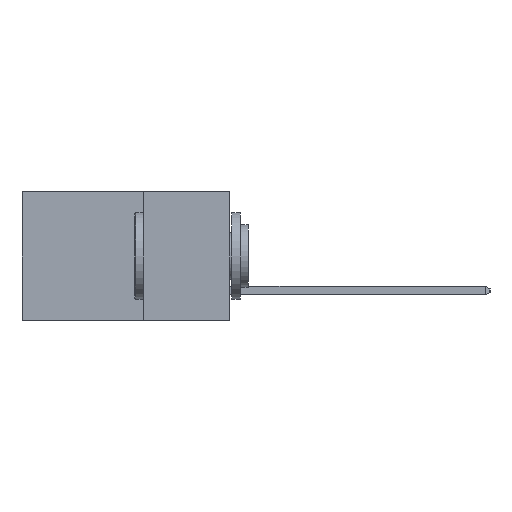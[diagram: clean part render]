
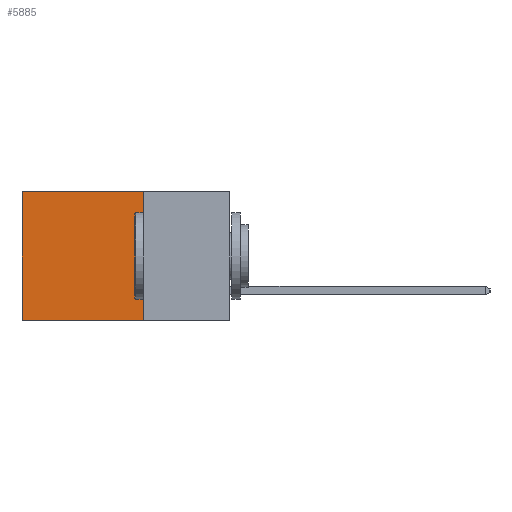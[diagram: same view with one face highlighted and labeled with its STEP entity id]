
A CAD part, left-side view. The second image highlights one B-rep face of the part: STEP entity #5885.
In plain terms, the highlighted planar face has unit normal (-1, 0, 0).
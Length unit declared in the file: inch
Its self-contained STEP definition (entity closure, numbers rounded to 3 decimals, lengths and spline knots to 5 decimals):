
#693 = CARTESIAN_POINT ( 'NONE',  ( 0.2615, 0.6, 0. ) ) ;
#1071 = LINE ( 'NONE', #3446, #3531 ) ;
#1847 = VERTEX_POINT ( 'NONE', #4616 ) ;
#3003 = VECTOR ( 'NONE', #11748, 39.37008 ) ;
#3446 = CARTESIAN_POINT ( 'NONE',  ( 0.2615, 0.6, -0.37 ) ) ;
#3531 = VECTOR ( 'NONE', #8729, 39.37008 ) ;
#3560 = VERTEX_POINT ( 'NONE', #10274 ) ;
#3584 = DIRECTION ( 'NONE',  ( 0., 0., -1. ) ) ;
#3601 = DIRECTION ( 'NONE',  ( 1., 0., 0. ) ) ;
#3747 = PLANE ( 'NONE',  #5497 ) ;
#3900 = VERTEX_POINT ( 'NONE', #5846 ) ;
#4072 = CARTESIAN_POINT ( 'NONE',  ( 0.2615, 0.25, -0.37 ) ) ;
#4321 = EDGE_CURVE ( 'NONE', #3560, #1847, #7819, .T. ) ;
#4616 = CARTESIAN_POINT ( 'NONE',  ( 0.2615, 0.25, -0.37 ) ) ;
#4629 = VERTEX_POINT ( 'NONE', #693 ) ;
#5127 = CARTESIAN_POINT ( 'NONE',  ( 0.2615, 0.25, -0.37 ) ) ;
#5398 = CARTESIAN_POINT ( 'NONE',  ( 0.2615, 0.25, 0. ) ) ;
#5497 = AXIS2_PLACEMENT_3D ( 'NONE', #4072, #3601, #3584 ) ;
#5514 = DIRECTION ( 'NONE',  ( 0., 0., -1. ) ) ;
#5825 = LINE ( 'NONE', #5398, #3003 ) ;
#5846 = CARTESIAN_POINT ( 'NONE',  ( 0.2615, 0.6, -0.37 ) ) ;
#5885 = ADVANCED_FACE ( 'NONE', ( #13101 ), #3747, .F. ) ;
#6139 = EDGE_CURVE ( 'NONE', #1847, #3900, #12314, .T. ) ;
#7819 = LINE ( 'NONE', #5127, #12994 ) ;
#8302 = ORIENTED_EDGE ( 'NONE', *, *, #4321, .F. ) ;
#8512 = EDGE_CURVE ( 'NONE', #3560, #4629, #5825, .T. ) ;
#8669 = ORIENTED_EDGE ( 'NONE', *, *, #8512, .T. ) ;
#8729 = DIRECTION ( 'NONE',  ( 0., 0., -1. ) ) ;
#9605 = VECTOR ( 'NONE', #11705, 39.37008 ) ;
#10274 = CARTESIAN_POINT ( 'NONE',  ( 0.2615, 0.25, 0. ) ) ;
#11564 = CARTESIAN_POINT ( 'NONE',  ( 0.2615, 0.25, -0.37 ) ) ;
#11705 = DIRECTION ( 'NONE',  ( 0., 1., 0. ) ) ;
#11748 = DIRECTION ( 'NONE',  ( 0., 1., 0. ) ) ;
#11828 = ORIENTED_EDGE ( 'NONE', *, *, #12776, .T. ) ;
#11976 = EDGE_LOOP ( 'NONE', ( #11828, #12753, #8302, #8669 ) ) ;
#12314 = LINE ( 'NONE', #11564, #9605 ) ;
#12753 = ORIENTED_EDGE ( 'NONE', *, *, #6139, .F. ) ;
#12776 = EDGE_CURVE ( 'NONE', #4629, #3900, #1071, .T. ) ;
#12994 = VECTOR ( 'NONE', #5514, 39.37008 ) ;
#13101 = FACE_OUTER_BOUND ( 'NONE', #11976, .T. ) ;
